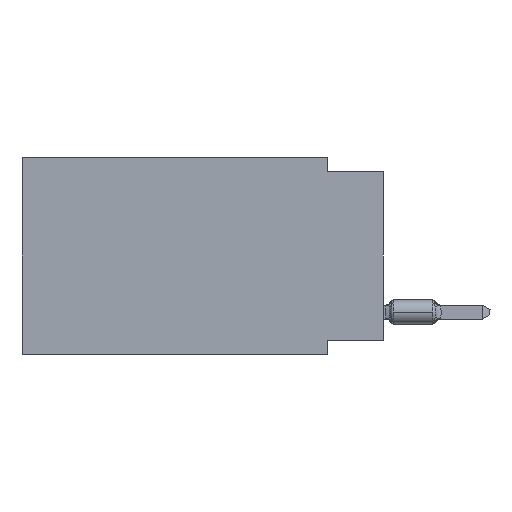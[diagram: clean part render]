
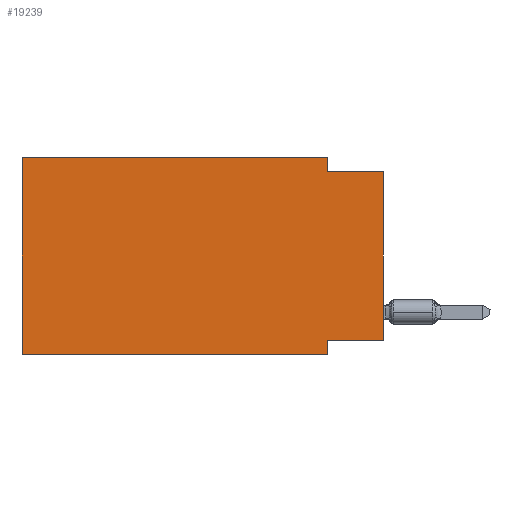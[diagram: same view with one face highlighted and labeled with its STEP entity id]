
A CAD part, left-side view. The second image highlights one B-rep face of the part: STEP entity #19239.
In plain terms, the highlighted planar face has unit normal (-1, 0, 0).
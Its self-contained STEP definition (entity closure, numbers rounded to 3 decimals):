
#278 = LINE ( 'NONE', #2992, #31202 ) ;
#313 = VERTEX_POINT ( 'NONE', #560 ) ;
#427 = DIRECTION ( 'NONE',  ( 0., -1., 0. ) ) ;
#560 = CARTESIAN_POINT ( 'NONE',  ( 0., 2.54, -8.89 ) ) ;
#642 = VECTOR ( 'NONE', #23076, 1000. ) ;
#830 = CARTESIAN_POINT ( 'NONE',  ( 0., 2.54, 0. ) ) ;
#1411 = ORIENTED_EDGE ( 'NONE', *, *, #7193, .F. ) ;
#2270 = ORIENTED_EDGE ( 'NONE', *, *, #22688, .F. ) ;
#2451 = EDGE_CURVE ( 'NONE', #30942, #5078, #11670, .T. ) ;
#2523 = CARTESIAN_POINT ( 'NONE',  ( 0., 16.383, -8.89 ) ) ;
#2992 = CARTESIAN_POINT ( 'NONE',  ( 0., 16.383, 0. ) ) ;
#4169 = LINE ( 'NONE', #22498, #18425 ) ;
#4382 = AXIS2_PLACEMENT_3D ( 'NONE', #9699, #17827, #20395 ) ;
#5078 = VERTEX_POINT ( 'NONE', #14234 ) ;
#5640 = EDGE_CURVE ( 'NONE', #19268, #21956, #9228, .T. ) ;
#6034 = VECTOR ( 'NONE', #22311, 1000. ) ;
#6386 = DIRECTION ( 'NONE',  ( 0., 0., 1. ) ) ;
#6549 = ORIENTED_EDGE ( 'NONE', *, *, #11779, .T. ) ;
#7111 = LINE ( 'NONE', #30358, #28266 ) ;
#7193 = EDGE_CURVE ( 'NONE', #10720, #13425, #278, .T. ) ;
#7269 = ORIENTED_EDGE ( 'NONE', *, *, #15695, .T. ) ;
#8114 = CARTESIAN_POINT ( 'NONE',  ( 0., 2.54, -8.255 ) ) ;
#9095 = LINE ( 'NONE', #27076, #19052 ) ;
#9219 = VECTOR ( 'NONE', #12840, 1000. ) ;
#9228 = LINE ( 'NONE', #19920, #6034 ) ;
#9650 = DIRECTION ( 'NONE',  ( 0., 0., -1. ) ) ;
#9676 = VERTEX_POINT ( 'NONE', #2523 ) ;
#9699 = CARTESIAN_POINT ( 'NONE',  ( 0., 16.383, 0. ) ) ;
#9839 = EDGE_CURVE ( 'NONE', #21956, #313, #7111, .T. ) ;
#10236 = CARTESIAN_POINT ( 'NONE',  ( 0., 16.383, 0. ) ) ;
#10720 = VERTEX_POINT ( 'NONE', #10236 ) ;
#11670 = LINE ( 'NONE', #22015, #9219 ) ;
#11779 = EDGE_CURVE ( 'NONE', #19268, #5078, #9095, .T. ) ;
#11955 = CARTESIAN_POINT ( 'NONE',  ( 0., 16.383, 0. ) ) ;
#12461 = LINE ( 'NONE', #11955, #24372 ) ;
#12840 = DIRECTION ( 'NONE',  ( 0., -1., 0. ) ) ;
#13425 = VERTEX_POINT ( 'NONE', #830 ) ;
#14234 = CARTESIAN_POINT ( 'NONE',  ( 0., 0., -0.635 ) ) ;
#15695 = EDGE_CURVE ( 'NONE', #9676, #313, #4169, .T. ) ;
#15772 = LINE ( 'NONE', #33596, #642 ) ;
#17809 = EDGE_LOOP ( 'NONE', ( #6549, #28556, #19185, #1411, #2270, #7269, #26998, #25989 ) ) ;
#17827 = DIRECTION ( 'NONE',  ( 1., 0., 0. ) ) ;
#18425 = VECTOR ( 'NONE', #27578, 1000. ) ;
#19052 = VECTOR ( 'NONE', #6386, 1000. ) ;
#19185 = ORIENTED_EDGE ( 'NONE', *, *, #27965, .F. ) ;
#19209 = FACE_OUTER_BOUND ( 'NONE', #17809, .T. ) ;
#19239 = ADVANCED_FACE ( 'NONE', ( #19209 ), #23103, .F. ) ;
#19268 = VERTEX_POINT ( 'NONE', #28200 ) ;
#19760 = CARTESIAN_POINT ( 'NONE',  ( 0., 2.54, -0.635 ) ) ;
#19920 = CARTESIAN_POINT ( 'NONE',  ( 0., 0., -8.255 ) ) ;
#20395 = DIRECTION ( 'NONE',  ( 0., 0., -1. ) ) ;
#21956 = VERTEX_POINT ( 'NONE', #8114 ) ;
#22015 = CARTESIAN_POINT ( 'NONE',  ( 0., 0., -0.635 ) ) ;
#22311 = DIRECTION ( 'NONE',  ( 0., 1., 0. ) ) ;
#22498 = CARTESIAN_POINT ( 'NONE',  ( 0., 16.383, -8.89 ) ) ;
#22688 = EDGE_CURVE ( 'NONE', #9676, #10720, #12461, .T. ) ;
#23076 = DIRECTION ( 'NONE',  ( 0., 0., -1. ) ) ;
#23103 = PLANE ( 'NONE',  #4382 ) ;
#24372 = VECTOR ( 'NONE', #27932, 1000. ) ;
#25989 = ORIENTED_EDGE ( 'NONE', *, *, #5640, .F. ) ;
#26998 = ORIENTED_EDGE ( 'NONE', *, *, #9839, .F. ) ;
#27076 = CARTESIAN_POINT ( 'NONE',  ( 0., 0., 0. ) ) ;
#27578 = DIRECTION ( 'NONE',  ( 0., -1., 0. ) ) ;
#27932 = DIRECTION ( 'NONE',  ( 0., 0., 1. ) ) ;
#27965 = EDGE_CURVE ( 'NONE', #13425, #30942, #15772, .T. ) ;
#28200 = CARTESIAN_POINT ( 'NONE',  ( 0., 0., -8.255 ) ) ;
#28266 = VECTOR ( 'NONE', #9650, 1000. ) ;
#28556 = ORIENTED_EDGE ( 'NONE', *, *, #2451, .F. ) ;
#30358 = CARTESIAN_POINT ( 'NONE',  ( 0., 2.54, -8.89 ) ) ;
#30942 = VERTEX_POINT ( 'NONE', #19760 ) ;
#31202 = VECTOR ( 'NONE', #427, 1000. ) ;
#33596 = CARTESIAN_POINT ( 'NONE',  ( 0., 2.54, 0. ) ) ;
